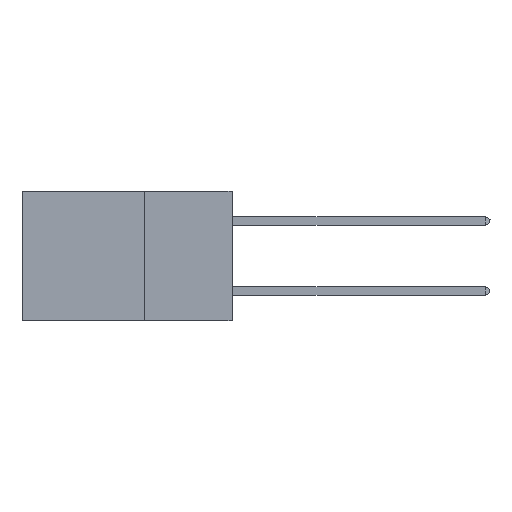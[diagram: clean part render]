
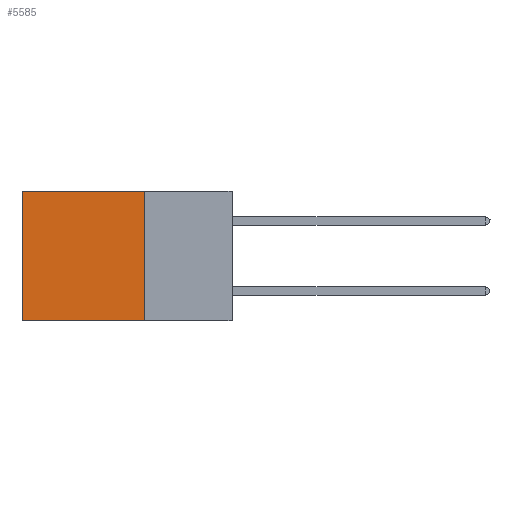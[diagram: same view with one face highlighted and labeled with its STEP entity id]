
A CAD part, left-side view. The second image highlights one B-rep face of the part: STEP entity #5585.
In plain terms, the highlighted planar face has unit normal (-1, 0, 0).
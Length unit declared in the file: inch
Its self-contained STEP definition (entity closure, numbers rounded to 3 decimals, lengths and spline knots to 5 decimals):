
#288 = CARTESIAN_POINT ( 'NONE',  ( 0.2875, 0.25, 0. ) ) ;
#527 = DIRECTION ( 'NONE',  ( 0., 1., 0. ) ) ;
#758 = VERTEX_POINT ( 'NONE', #4560 ) ;
#1080 = ORIENTED_EDGE ( 'NONE', *, *, #14722, .T. ) ;
#1376 = VECTOR ( 'NONE', #5075, 39.37008 ) ;
#1676 = DIRECTION ( 'NONE',  ( 1., 0., 0. ) ) ;
#2016 = CARTESIAN_POINT ( 'NONE',  ( 0.2875, 0.6, -0.37 ) ) ;
#3465 = FACE_OUTER_BOUND ( 'NONE', #9663, .T. ) ;
#3770 = CARTESIAN_POINT ( 'NONE',  ( 0.2875, 0.25, 0. ) ) ;
#4560 = CARTESIAN_POINT ( 'NONE',  ( 0.2875, 0.6, 0. ) ) ;
#4605 = EDGE_CURVE ( 'NONE', #12859, #758, #5170, .T. ) ;
#4749 = LINE ( 'NONE', #8725, #1376 ) ;
#5075 = DIRECTION ( 'NONE',  ( 0., 0., -1. ) ) ;
#5170 = LINE ( 'NONE', #13377, #7666 ) ;
#5585 = ADVANCED_FACE ( 'NONE', ( #3465 ), #7867, .F. ) ;
#5711 = ORIENTED_EDGE ( 'NONE', *, *, #9780, .F. ) ;
#6633 = VECTOR ( 'NONE', #527, 39.37008 ) ;
#7666 = VECTOR ( 'NONE', #14558, 39.37008 ) ;
#7708 = ORIENTED_EDGE ( 'NONE', *, *, #15015, .F. ) ;
#7867 = PLANE ( 'NONE',  #15737 ) ;
#8162 = CARTESIAN_POINT ( 'NONE',  ( 0.2875, 0.25, -0.37 ) ) ;
#8725 = CARTESIAN_POINT ( 'NONE',  ( 0.2875, 0.6, 0. ) ) ;
#9363 = DIRECTION ( 'NONE',  ( 0., 0., -1. ) ) ;
#9663 = EDGE_LOOP ( 'NONE', ( #1080, #7708, #5711, #10839 ) ) ;
#9780 = EDGE_CURVE ( 'NONE', #12859, #15736, #10197, .T. ) ;
#10197 = LINE ( 'NONE', #11771, #13025 ) ;
#10313 = DIRECTION ( 'NONE',  ( 0., 0., -1. ) ) ;
#10839 = ORIENTED_EDGE ( 'NONE', *, *, #4605, .T. ) ;
#11652 = CARTESIAN_POINT ( 'NONE',  ( 0.2875, 0.25, -0.37 ) ) ;
#11771 = CARTESIAN_POINT ( 'NONE',  ( 0.2875, 0.25, 0. ) ) ;
#12859 = VERTEX_POINT ( 'NONE', #3770 ) ;
#13025 = VECTOR ( 'NONE', #9363, 39.37008 ) ;
#13096 = LINE ( 'NONE', #11652, #6633 ) ;
#13377 = CARTESIAN_POINT ( 'NONE',  ( 0.2875, 0.25, 0. ) ) ;
#14558 = DIRECTION ( 'NONE',  ( 0., 1., 0. ) ) ;
#14722 = EDGE_CURVE ( 'NONE', #758, #15078, #4749, .T. ) ;
#15015 = EDGE_CURVE ( 'NONE', #15736, #15078, #13096, .T. ) ;
#15078 = VERTEX_POINT ( 'NONE', #2016 ) ;
#15736 = VERTEX_POINT ( 'NONE', #8162 ) ;
#15737 = AXIS2_PLACEMENT_3D ( 'NONE', #288, #1676, #10313 ) ;
